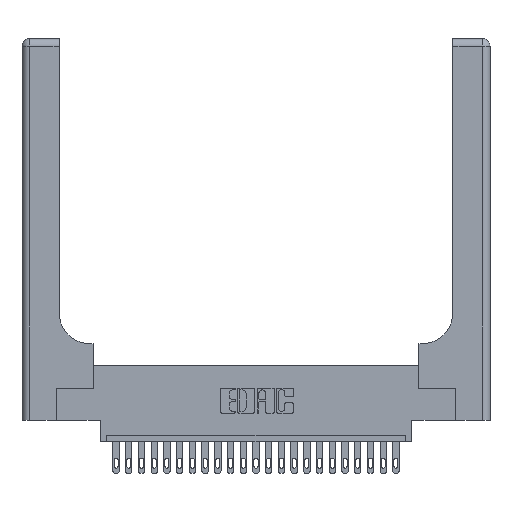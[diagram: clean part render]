
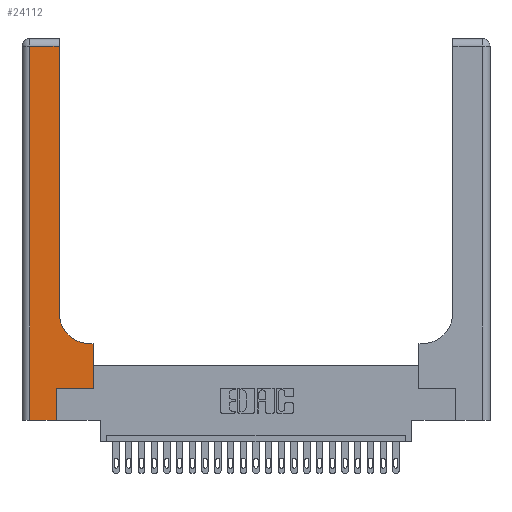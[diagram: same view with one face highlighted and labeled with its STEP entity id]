
A CAD part, top view. The second image highlights one B-rep face of the part: STEP entity #24112.
In plain terms, the highlighted planar face has unit normal (0, 0, 1).
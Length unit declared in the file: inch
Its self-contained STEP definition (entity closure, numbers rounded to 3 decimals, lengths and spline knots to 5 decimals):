
#326 = LINE ( 'NONE', #16498, #4225 ) ;
#425 = LINE ( 'NONE', #7420, #6796 ) ;
#689 = LINE ( 'NONE', #20767, #4311 ) ;
#701 = CARTESIAN_POINT ( 'NONE',  ( 0.269, 0., 0.37 ) ) ;
#1012 = ORIENTED_EDGE ( 'NONE', *, *, #2803, .T. ) ;
#1094 = CARTESIAN_POINT ( 'NONE',  ( 0.269, 0.25, 0.37 ) ) ;
#1154 = VERTEX_POINT ( 'NONE', #20155 ) ;
#1377 = CARTESIAN_POINT ( 'NONE',  ( 0.2915, 2.94, 0.37 ) ) ;
#2064 = CARTESIAN_POINT ( 'NONE',  ( 0.269, 0.25, 0.37 ) ) ;
#2115 = VERTEX_POINT ( 'NONE', #23357 ) ;
#2298 = VERTEX_POINT ( 'NONE', #21196 ) ;
#2575 = VERTEX_POINT ( 'NONE', #20324 ) ;
#2803 = EDGE_CURVE ( 'NONE', #2115, #3729, #326, .T. ) ;
#2810 = DIRECTION ( 'NONE',  ( 0., 0., -1. ) ) ;
#2881 = VERTEX_POINT ( 'NONE', #18656 ) ;
#3708 = DIRECTION ( 'NONE',  ( 0., 0., -1. ) ) ;
#3729 = VERTEX_POINT ( 'NONE', #701 ) ;
#4103 = EDGE_CURVE ( 'NONE', #2881, #15061, #13605, .T. ) ;
#4225 = VECTOR ( 'NONE', #16579, 39.37008 ) ;
#4311 = VECTOR ( 'NONE', #17034, 39.37008 ) ;
#4717 = CARTESIAN_POINT ( 'NONE',  ( 0.269, 0., 0.37 ) ) ;
#6394 = ORIENTED_EDGE ( 'NONE', *, *, #10896, .T. ) ;
#6519 = ORIENTED_EDGE ( 'NONE', *, *, #11537, .T. ) ;
#6729 = LINE ( 'NONE', #4717, #17640 ) ;
#6796 = VECTOR ( 'NONE', #13131, 39.37008 ) ;
#7113 = EDGE_LOOP ( 'NONE', ( #9794, #18144, #6394, #1012, #21215, #24114, #7999, #20710, #6519 ) ) ;
#7420 = CARTESIAN_POINT ( 'NONE',  ( 0.5585, 0.25, 0.37 ) ) ;
#7999 = ORIENTED_EDGE ( 'NONE', *, *, #17979, .T. ) ;
#8288 = DIRECTION ( 'NONE',  ( 0., 1., 0. ) ) ;
#8811 = LINE ( 'NONE', #21513, #22459 ) ;
#9571 = EDGE_CURVE ( 'NONE', #17630, #2575, #689, .T. ) ;
#9647 = VECTOR ( 'NONE', #13841, 39.37008 ) ;
#9794 = ORIENTED_EDGE ( 'NONE', *, *, #11088, .T. ) ;
#10252 = EDGE_CURVE ( 'NONE', #3729, #10943, #6729, .T. ) ;
#10804 = CARTESIAN_POINT ( 'NONE',  ( 0., 3., 0.37 ) ) ;
#10896 = EDGE_CURVE ( 'NONE', #2575, #2115, #17588, .T. ) ;
#10943 = VERTEX_POINT ( 'NONE', #1094 ) ;
#11088 = EDGE_CURVE ( 'NONE', #2298, #17630, #8811, .T. ) ;
#11537 = EDGE_CURVE ( 'NONE', #15061, #2298, #13932, .T. ) ;
#12585 = DIRECTION ( 'NONE',  ( 0., -1., 0. ) ) ;
#12673 = PLANE ( 'NONE',  #21958 ) ;
#13131 = DIRECTION ( 'NONE',  ( 0., 1., 0. ) ) ;
#13312 = FACE_OUTER_BOUND ( 'NONE', #7113, .T. ) ;
#13359 = VECTOR ( 'NONE', #12585, 39.37008 ) ;
#13605 = LINE ( 'NONE', #19619, #9647 ) ;
#13841 = DIRECTION ( 'NONE',  ( -1., 0., 0. ) ) ;
#13932 = CIRCLE ( 'NONE', #19255, 0.25 ) ;
#14221 = CARTESIAN_POINT ( 'NONE',  ( 0.5415, 0.6, 0.37 ) ) ;
#14273 = CARTESIAN_POINT ( 'NONE',  ( 0.06, 3., 0.37 ) ) ;
#14685 = DIRECTION ( 'NONE',  ( 1., 0., 0. ) ) ;
#15061 = VERTEX_POINT ( 'NONE', #14221 ) ;
#16027 = DIRECTION ( 'NONE',  ( 0., 1., 0. ) ) ;
#16328 = DIRECTION ( 'NONE',  ( -1., 0., 0. ) ) ;
#16498 = CARTESIAN_POINT ( 'NONE',  ( 0., 0., 0.37 ) ) ;
#16579 = DIRECTION ( 'NONE',  ( 1., 0., 0. ) ) ;
#16984 = CARTESIAN_POINT ( 'NONE',  ( 0.5415, 0.85, 0.37 ) ) ;
#17034 = DIRECTION ( 'NONE',  ( -1., 0., 0. ) ) ;
#17231 = DIRECTION ( 'NONE',  ( 1., 0., 0. ) ) ;
#17588 = LINE ( 'NONE', #14273, #13359 ) ;
#17630 = VERTEX_POINT ( 'NONE', #1377 ) ;
#17640 = VECTOR ( 'NONE', #8288, 39.37008 ) ;
#17979 = EDGE_CURVE ( 'NONE', #1154, #2881, #425, .T. ) ;
#18007 = LINE ( 'NONE', #2064, #22547 ) ;
#18144 = ORIENTED_EDGE ( 'NONE', *, *, #9571, .T. ) ;
#18656 = CARTESIAN_POINT ( 'NONE',  ( 0.5585, 0.6, 0.37 ) ) ;
#19255 = AXIS2_PLACEMENT_3D ( 'NONE', #16984, #3708, #17231 ) ;
#19619 = CARTESIAN_POINT ( 'NONE',  ( 0.2915, 0.6, 0.37 ) ) ;
#20155 = CARTESIAN_POINT ( 'NONE',  ( 0.5585, 0.25, 0.37 ) ) ;
#20324 = CARTESIAN_POINT ( 'NONE',  ( 0.06, 2.94, 0.37 ) ) ;
#20710 = ORIENTED_EDGE ( 'NONE', *, *, #4103, .T. ) ;
#20767 = CARTESIAN_POINT ( 'NONE',  ( 0., 2.94, 0.37 ) ) ;
#20975 = EDGE_CURVE ( 'NONE', #10943, #1154, #18007, .T. ) ;
#21196 = CARTESIAN_POINT ( 'NONE',  ( 0.2915, 0.85, 0.37 ) ) ;
#21215 = ORIENTED_EDGE ( 'NONE', *, *, #10252, .T. ) ;
#21513 = CARTESIAN_POINT ( 'NONE',  ( 0.2915, 3., 0.37 ) ) ;
#21958 = AXIS2_PLACEMENT_3D ( 'NONE', #10804, #2810, #16328 ) ;
#22459 = VECTOR ( 'NONE', #16027, 39.37008 ) ;
#22547 = VECTOR ( 'NONE', #14685, 39.37008 ) ;
#23357 = CARTESIAN_POINT ( 'NONE',  ( 0.06, 0., 0.37 ) ) ;
#24112 = ADVANCED_FACE ( 'NONE', ( #13312 ), #12673, .F. ) ;
#24114 = ORIENTED_EDGE ( 'NONE', *, *, #20975, .T. ) ;
